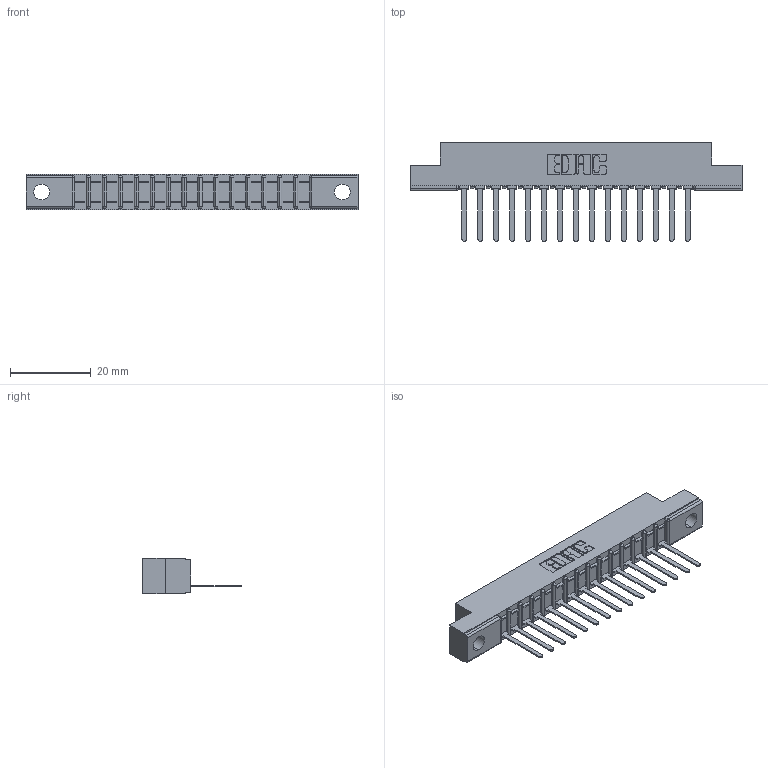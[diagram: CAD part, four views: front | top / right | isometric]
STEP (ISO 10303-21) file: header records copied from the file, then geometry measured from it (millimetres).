
FILE_DESCRIPTION (( 'STEP AP203' ), '1' );
FILE_NAME ('357-015-441-104.STEP', '2020-09-30T17:56:28', ( '' ), ( '' ), 'SwSTEP 2.0', 'SolidWorks 2020', '' );
FILE_SCHEMA (( 'CONFIG_CONTROL_DESIGN' ));
Length unit declared in the file: inch
Products named in the file (3): 357-015-441-104; 307 Part_.156 Dia Mounting Holes; 307-290-002_541
Assembly tree (16 placements, depth 2):
  357-015-441-104
    307 Part_.156 Dia Mounting Holes
    307-290-002_541  x15
Bounding box: 82.45 x 24.59 x 8.71 mm (x, y, z)
Volume: 5375.8 mm3; surface area: 9534.8 mm2
Topology: 16 solids, 16 shells, 1258 faces, 3839 edges, 2514 vertices
Faces by surface type: plane 759, cylinder 467, sphere 32
Entity records: 17324 total; most frequent: CARTESIAN_POINT 2922, ORIENTED_EDGE 2910, DIRECTION 2843, EDGE_CURVE 1455, VECTOR 1109, LINE 1109, VERTEX_POINT 946, AXIS2_PLACEMENT_3D 867
